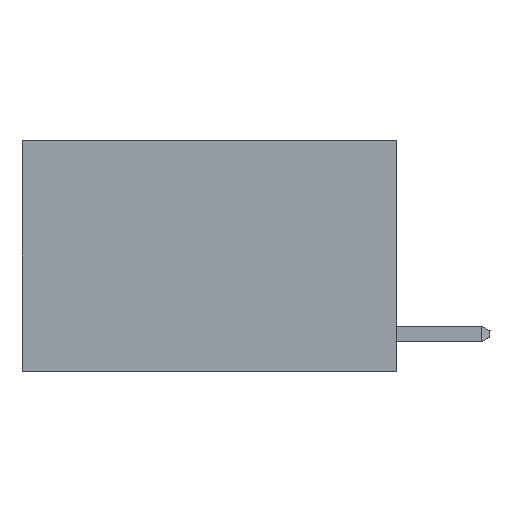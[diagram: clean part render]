
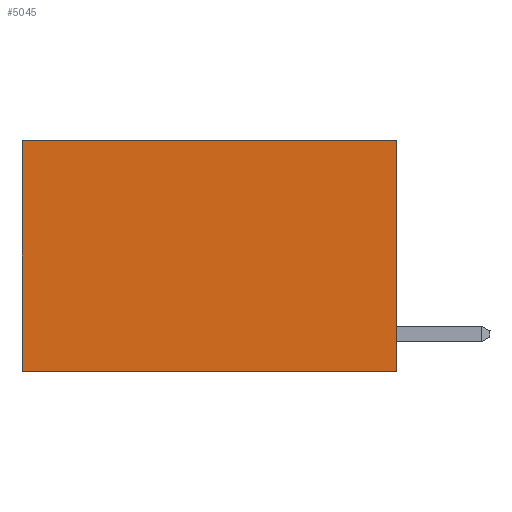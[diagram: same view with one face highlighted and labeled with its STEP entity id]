
A CAD part, left-side view. The second image highlights one B-rep face of the part: STEP entity #5045.
In plain terms, the highlighted planar face has unit normal (-1, 0, 0).
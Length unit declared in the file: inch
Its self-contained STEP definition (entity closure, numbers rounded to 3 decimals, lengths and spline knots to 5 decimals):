
#396 = CARTESIAN_POINT ( 'NONE',  ( 0.2625, 0., 0. ) ) ;
#747 = EDGE_CURVE ( 'NONE', #18988, #16257, #16889, .T. ) ;
#831 = DIRECTION ( 'NONE',  ( 0., 0., -1. ) ) ;
#860 = VECTOR ( 'NONE', #9161, 39.37008 ) ;
#900 = DIRECTION ( 'NONE',  ( 0., 1., 0. ) ) ;
#1636 = CARTESIAN_POINT ( 'NONE',  ( 0.2625, 0.6, 0. ) ) ;
#3208 = VECTOR ( 'NONE', #10741, 39.37008 ) ;
#3410 = VECTOR ( 'NONE', #900, 39.37008 ) ;
#3819 = LINE ( 'NONE', #23997, #3208 ) ;
#4219 = ORIENTED_EDGE ( 'NONE', *, *, #7194, .F. ) ;
#5045 = ADVANCED_FACE ( 'NONE', ( #7131 ), #8614, .F. ) ;
#6013 = ORIENTED_EDGE ( 'NONE', *, *, #23545, .T. ) ;
#7131 = FACE_OUTER_BOUND ( 'NONE', #18375, .T. ) ;
#7194 = EDGE_CURVE ( 'NONE', #16257, #20212, #3819, .T. ) ;
#7749 = CARTESIAN_POINT ( 'NONE',  ( 0.2625, 0.6, 0. ) ) ;
#8322 = CARTESIAN_POINT ( 'NONE',  ( 0.2625, 0.6, -0.37 ) ) ;
#8614 = PLANE ( 'NONE',  #23439 ) ;
#9161 = DIRECTION ( 'NONE',  ( 0., 0., -1. ) ) ;
#9598 = EDGE_CURVE ( 'NONE', #18988, #20538, #13042, .T. ) ;
#10741 = DIRECTION ( 'NONE',  ( 0., 1., 0. ) ) ;
#12465 = DIRECTION ( 'NONE',  ( 1., 0., 0. ) ) ;
#12530 = CARTESIAN_POINT ( 'NONE',  ( 0.2625, 0., 0. ) ) ;
#13042 = LINE ( 'NONE', #12530, #3410 ) ;
#14731 = VECTOR ( 'NONE', #21055, 39.37008 ) ;
#14803 = ORIENTED_EDGE ( 'NONE', *, *, #747, .F. ) ;
#15338 = LINE ( 'NONE', #7749, #14731 ) ;
#15651 = CARTESIAN_POINT ( 'NONE',  ( 0.2625, 0., -0.37 ) ) ;
#16257 = VERTEX_POINT ( 'NONE', #15651 ) ;
#16889 = LINE ( 'NONE', #18548, #860 ) ;
#18375 = EDGE_LOOP ( 'NONE', ( #6013, #4219, #14803, #23986 ) ) ;
#18548 = CARTESIAN_POINT ( 'NONE',  ( 0.2625, 0., 0. ) ) ;
#18988 = VERTEX_POINT ( 'NONE', #396 ) ;
#20212 = VERTEX_POINT ( 'NONE', #8322 ) ;
#20538 = VERTEX_POINT ( 'NONE', #1636 ) ;
#21055 = DIRECTION ( 'NONE',  ( 0., 0., -1. ) ) ;
#23439 = AXIS2_PLACEMENT_3D ( 'NONE', #23792, #12465, #831 ) ;
#23545 = EDGE_CURVE ( 'NONE', #20538, #20212, #15338, .T. ) ;
#23792 = CARTESIAN_POINT ( 'NONE',  ( 0.2625, 0., 0. ) ) ;
#23986 = ORIENTED_EDGE ( 'NONE', *, *, #9598, .T. ) ;
#23997 = CARTESIAN_POINT ( 'NONE',  ( 0.2625, 0., -0.37 ) ) ;
